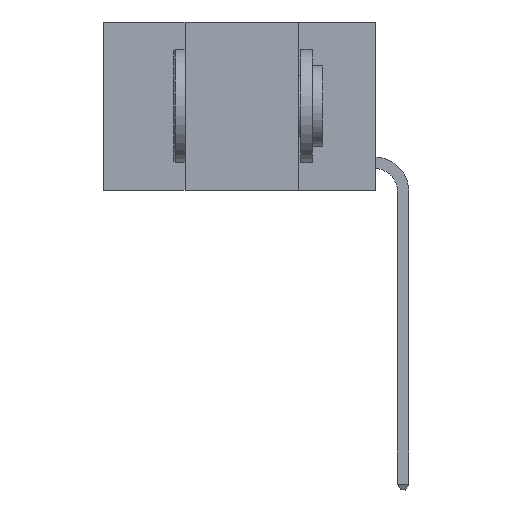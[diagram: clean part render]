
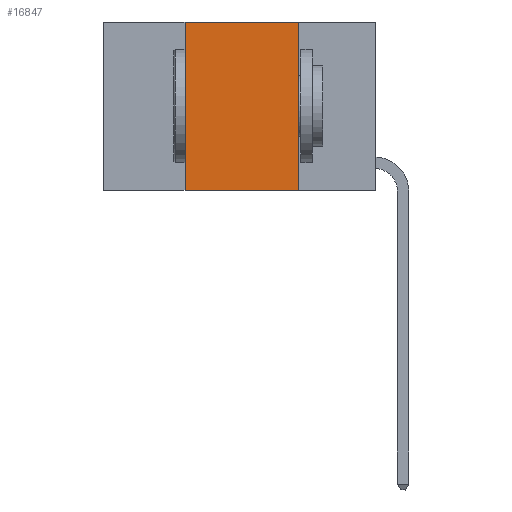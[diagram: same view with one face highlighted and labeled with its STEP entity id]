
A CAD part, left-side view. The second image highlights one B-rep face of the part: STEP entity #16847.
In plain terms, the highlighted planar face has unit normal (-1, 0, 0).
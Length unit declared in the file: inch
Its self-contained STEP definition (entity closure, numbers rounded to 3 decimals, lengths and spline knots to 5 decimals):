
#286 = VERTEX_POINT ( 'NONE', #12856 ) ;
#649 = EDGE_CURVE ( 'NONE', #6507, #286, #9023, .T. ) ;
#812 = VERTEX_POINT ( 'NONE', #6725 ) ;
#852 = DIRECTION ( 'NONE',  ( 0., 0., 1. ) ) ;
#866 = VECTOR ( 'NONE', #18553, 39.37008 ) ;
#3040 = FACE_OUTER_BOUND ( 'NONE', #15805, .T. ) ;
#5477 = VERTEX_POINT ( 'NONE', #21487 ) ;
#5828 = LINE ( 'NONE', #18473, #866 ) ;
#6080 = CARTESIAN_POINT ( 'NONE',  ( 0., 0.42, 0. ) ) ;
#6507 = VERTEX_POINT ( 'NONE', #6080 ) ;
#6632 = EDGE_CURVE ( 'NONE', #812, #6507, #23225, .T. ) ;
#6666 = VECTOR ( 'NONE', #21435, 39.37008 ) ;
#6725 = CARTESIAN_POINT ( 'NONE',  ( 0., 0.42, -0.37 ) ) ;
#8260 = CARTESIAN_POINT ( 'NONE',  ( 0., 0.42, 0. ) ) ;
#8670 = CARTESIAN_POINT ( 'NONE',  ( 0., 0.6, 0. ) ) ;
#9023 = LINE ( 'NONE', #9998, #22793 ) ;
#9239 = EDGE_CURVE ( 'NONE', #812, #5477, #5828, .T. ) ;
#9998 = CARTESIAN_POINT ( 'NONE',  ( 0., 0.6, 0. ) ) ;
#10480 = DIRECTION ( 'NONE',  ( 0., 0., -1. ) ) ;
#12028 = LINE ( 'NONE', #23182, #6666 ) ;
#12184 = PLANE ( 'NONE',  #14513 ) ;
#12204 = DIRECTION ( 'NONE',  ( 0., -1., 0. ) ) ;
#12856 = CARTESIAN_POINT ( 'NONE',  ( 0., 0.17, 0. ) ) ;
#14513 = AXIS2_PLACEMENT_3D ( 'NONE', #8670, #21295, #10480 ) ;
#15402 = EDGE_CURVE ( 'NONE', #286, #5477, #12028, .T. ) ;
#15457 = ORIENTED_EDGE ( 'NONE', *, *, #15402, .F. ) ;
#15805 = EDGE_LOOP ( 'NONE', ( #15457, #15853, #16288, #17579 ) ) ;
#15853 = ORIENTED_EDGE ( 'NONE', *, *, #649, .F. ) ;
#16288 = ORIENTED_EDGE ( 'NONE', *, *, #6632, .F. ) ;
#16847 = ADVANCED_FACE ( 'NONE', ( #3040 ), #12184, .F. ) ;
#17579 = ORIENTED_EDGE ( 'NONE', *, *, #9239, .T. ) ;
#18473 = CARTESIAN_POINT ( 'NONE',  ( 0., 0.6, -0.37 ) ) ;
#18501 = VECTOR ( 'NONE', #852, 39.37008 ) ;
#18553 = DIRECTION ( 'NONE',  ( 0., -1., 0. ) ) ;
#21295 = DIRECTION ( 'NONE',  ( 1., 0., 0. ) ) ;
#21435 = DIRECTION ( 'NONE',  ( 0., 0., -1. ) ) ;
#21487 = CARTESIAN_POINT ( 'NONE',  ( 0., 0.17, -0.37 ) ) ;
#22793 = VECTOR ( 'NONE', #12204, 39.37008 ) ;
#23182 = CARTESIAN_POINT ( 'NONE',  ( 0., 0.17, 0. ) ) ;
#23225 = LINE ( 'NONE', #8260, #18501 ) ;
